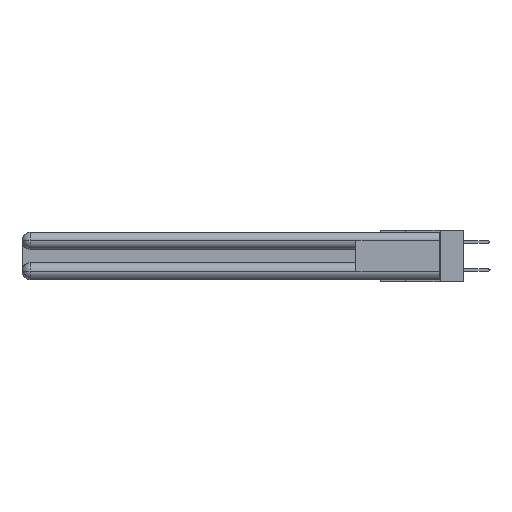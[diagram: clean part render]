
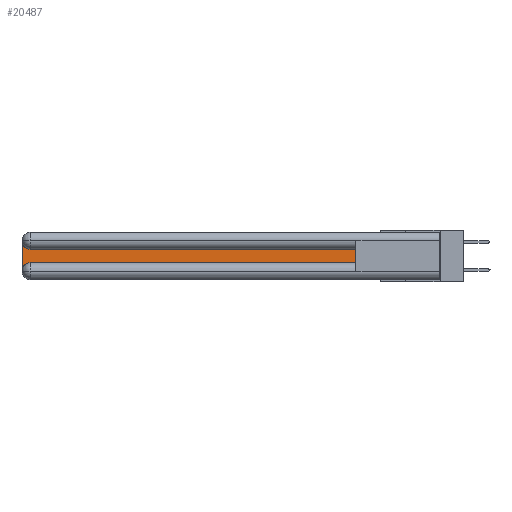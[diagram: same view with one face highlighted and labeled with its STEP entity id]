
A CAD part, left-side view. The second image highlights one B-rep face of the part: STEP entity #20487.
In plain terms, the highlighted planar face has unit normal (-1, 0, 0).
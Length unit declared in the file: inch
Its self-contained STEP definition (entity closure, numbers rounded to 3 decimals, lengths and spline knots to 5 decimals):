
#356 = VECTOR ( 'NONE', #8077, 39.37008 ) ;
#360 = DIRECTION ( 'NONE',  ( 1., 0., 0. ) ) ;
#509 = VECTOR ( 'NONE', #12772, 39.37008 ) ;
#898 = EDGE_CURVE ( 'NONE', #19670, #25104, #27224, .T. ) ;
#1438 = AXIS2_PLACEMENT_3D ( 'NONE', #29533, #13748, #16512 ) ;
#3025 = DIRECTION ( 'NONE',  ( 0., 0., -1. ) ) ;
#4677 = ORIENTED_EDGE ( 'NONE', *, *, #18485, .T. ) ;
#4708 = ORIENTED_EDGE ( 'NONE', *, *, #19208, .T. ) ;
#5782 = ORIENTED_EDGE ( 'NONE', *, *, #6061, .T. ) ;
#6061 = EDGE_CURVE ( 'NONE', #8435, #23318, #26480, .T. ) ;
#6159 = CIRCLE ( 'NONE', #28240, 0.06 ) ;
#6516 = EDGE_CURVE ( 'NONE', #23846, #8435, #6159, .T. ) ;
#7495 = CARTESIAN_POINT ( 'NONE',  ( 0.075, 2.94, -0.2175 ) ) ;
#8033 = ORIENTED_EDGE ( 'NONE', *, *, #31784, .T. ) ;
#8077 = DIRECTION ( 'NONE',  ( 0., 0., 1. ) ) ;
#8435 = VERTEX_POINT ( 'NONE', #12829 ) ;
#8576 = ORIENTED_EDGE ( 'NONE', *, *, #6516, .T. ) ;
#8600 = CARTESIAN_POINT ( 'NONE',  ( 0.075, 3., -0.2175 ) ) ;
#10393 = CARTESIAN_POINT ( 'NONE',  ( 0.075, 0.6, -0.2175 ) ) ;
#12772 = DIRECTION ( 'NONE',  ( 0., -1., 0. ) ) ;
#12829 = CARTESIAN_POINT ( 'NONE',  ( 0.075, 3., -0.0625 ) ) ;
#12979 = CARTESIAN_POINT ( 'NONE',  ( 0.075, 0.6, -0.2175 ) ) ;
#13534 = DIRECTION ( 'NONE',  ( 0., 0., -1. ) ) ;
#13748 = DIRECTION ( 'NONE',  ( 1., 0., 0. ) ) ;
#14336 = CARTESIAN_POINT ( 'NONE',  ( 0.075, 3., -0.2775 ) ) ;
#14589 = LINE ( 'NONE', #15222, #509 ) ;
#15171 = ORIENTED_EDGE ( 'NONE', *, *, #898, .T. ) ;
#15222 = CARTESIAN_POINT ( 'NONE',  ( 0.075, 0.6, -0.2175 ) ) ;
#15340 = LINE ( 'NONE', #28546, #16180 ) ;
#15624 = DIRECTION ( 'NONE',  ( 0., 1., 0. ) ) ;
#15933 = FACE_OUTER_BOUND ( 'NONE', #20971, .T. ) ;
#16024 = VERTEX_POINT ( 'NONE', #7495 ) ;
#16180 = VECTOR ( 'NONE', #15624, 39.37008 ) ;
#16512 = DIRECTION ( 'NONE',  ( 0., 0., -1. ) ) ;
#16600 = CARTESIAN_POINT ( 'NONE',  ( 0.075, 2.94, -0.1225 ) ) ;
#18142 = DIRECTION ( 'NONE',  ( 1., 0., 0. ) ) ;
#18485 = EDGE_CURVE ( 'NONE', #16024, #19670, #14589, .T. ) ;
#19208 = EDGE_CURVE ( 'NONE', #25104, #23846, #15340, .T. ) ;
#19670 = VERTEX_POINT ( 'NONE', #12979 ) ;
#20487 = ADVANCED_FACE ( 'NONE', ( #15933 ), #26829, .F. ) ;
#20802 = DIRECTION ( 'NONE',  ( 0., 0., -1. ) ) ;
#20971 = EDGE_LOOP ( 'NONE', ( #4708, #8576, #5782, #8033, #4677, #15171 ) ) ;
#22713 = CARTESIAN_POINT ( 'NONE',  ( 0.075, 0.6, -0.1225 ) ) ;
#23318 = VERTEX_POINT ( 'NONE', #14336 ) ;
#23846 = VERTEX_POINT ( 'NONE', #16600 ) ;
#25104 = VERTEX_POINT ( 'NONE', #22713 ) ;
#25989 = CARTESIAN_POINT ( 'NONE',  ( 0.075, 2.94, -0.0625 ) ) ;
#26480 = LINE ( 'NONE', #8600, #31391 ) ;
#26829 = PLANE ( 'NONE',  #27363 ) ;
#27224 = LINE ( 'NONE', #10393, #356 ) ;
#27363 = AXIS2_PLACEMENT_3D ( 'NONE', #31523, #360, #13534 ) ;
#28240 = AXIS2_PLACEMENT_3D ( 'NONE', #25989, #18142, #20802 ) ;
#28357 = CIRCLE ( 'NONE', #1438, 0.06 ) ;
#28546 = CARTESIAN_POINT ( 'NONE',  ( 0.075, 0.6, -0.1225 ) ) ;
#29533 = CARTESIAN_POINT ( 'NONE',  ( 0.075, 2.94, -0.2775 ) ) ;
#31391 = VECTOR ( 'NONE', #3025, 39.37008 ) ;
#31523 = CARTESIAN_POINT ( 'NONE',  ( 0.075, 3., -0.1225 ) ) ;
#31784 = EDGE_CURVE ( 'NONE', #23318, #16024, #28357, .T. ) ;
